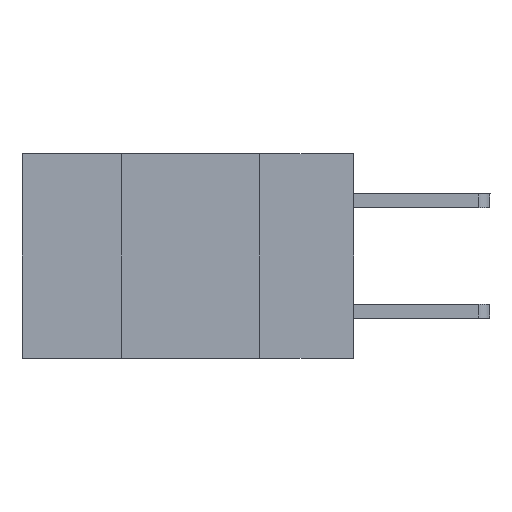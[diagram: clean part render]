
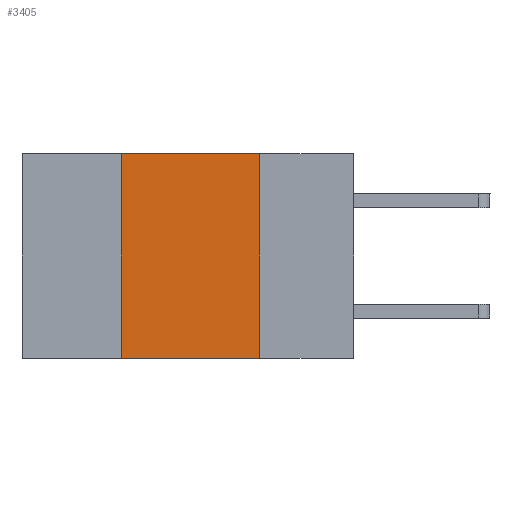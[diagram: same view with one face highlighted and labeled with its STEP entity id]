
A CAD part, left-side view. The second image highlights one B-rep face of the part: STEP entity #3405.
In plain terms, the highlighted planar face has unit normal (-1, 0, 0).
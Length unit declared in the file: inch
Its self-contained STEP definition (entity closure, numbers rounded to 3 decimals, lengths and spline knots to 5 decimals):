
#118 = EDGE_CURVE ( 'NONE', #2263, #1840, #2727, .T. ) ;
#458 = EDGE_CURVE ( 'NONE', #1840, #5806, #6440, .T. ) ;
#470 = CARTESIAN_POINT ( 'NONE',  ( 0., 0.42, -0.37 ) ) ;
#482 = DIRECTION ( 'NONE',  ( 0., 0., -1. ) ) ;
#914 = ORIENTED_EDGE ( 'NONE', *, *, #118, .F. ) ;
#1840 = VERTEX_POINT ( 'NONE', #5349 ) ;
#2181 = CARTESIAN_POINT ( 'NONE',  ( 0., 0.6, 0. ) ) ;
#2190 = ORIENTED_EDGE ( 'NONE', *, *, #10138, .T. ) ;
#2263 = VERTEX_POINT ( 'NONE', #5125 ) ;
#2301 = VECTOR ( 'NONE', #12396, 39.37008 ) ;
#2376 = ORIENTED_EDGE ( 'NONE', *, *, #9378, .F. ) ;
#2727 = LINE ( 'NONE', #11437, #2301 ) ;
#2927 = DIRECTION ( 'NONE',  ( 0., 0., -1. ) ) ;
#3405 = ADVANCED_FACE ( 'NONE', ( #5164 ), #8704, .F. ) ;
#4052 = VERTEX_POINT ( 'NONE', #470 ) ;
#4908 = DIRECTION ( 'NONE',  ( 1., 0., 0. ) ) ;
#5125 = CARTESIAN_POINT ( 'NONE',  ( 0., 0.42, 0. ) ) ;
#5164 = FACE_OUTER_BOUND ( 'NONE', #12755, .T. ) ;
#5349 = CARTESIAN_POINT ( 'NONE',  ( 0., 0.17, 0. ) ) ;
#5586 = DIRECTION ( 'NONE',  ( 0., -1., 0. ) ) ;
#5806 = VERTEX_POINT ( 'NONE', #5840 ) ;
#5808 = VECTOR ( 'NONE', #482, 39.37008 ) ;
#5815 = DIRECTION ( 'NONE',  ( 0., 0., 1. ) ) ;
#5840 = CARTESIAN_POINT ( 'NONE',  ( 0., 0.17, -0.37 ) ) ;
#6390 = VECTOR ( 'NONE', #5586, 39.37008 ) ;
#6440 = LINE ( 'NONE', #9325, #5808 ) ;
#6509 = CARTESIAN_POINT ( 'NONE',  ( 0., 0.6, -0.37 ) ) ;
#7633 = AXIS2_PLACEMENT_3D ( 'NONE', #2181, #4908, #2927 ) ;
#7977 = ORIENTED_EDGE ( 'NONE', *, *, #458, .F. ) ;
#8704 = PLANE ( 'NONE',  #7633 ) ;
#9325 = CARTESIAN_POINT ( 'NONE',  ( 0., 0.17, 0. ) ) ;
#9378 = EDGE_CURVE ( 'NONE', #4052, #2263, #12577, .T. ) ;
#9635 = CARTESIAN_POINT ( 'NONE',  ( 0., 0.42, 0. ) ) ;
#10138 = EDGE_CURVE ( 'NONE', #4052, #5806, #11641, .T. ) ;
#10887 = VECTOR ( 'NONE', #5815, 39.37008 ) ;
#11437 = CARTESIAN_POINT ( 'NONE',  ( 0., 0.6, 0. ) ) ;
#11641 = LINE ( 'NONE', #6509, #6390 ) ;
#12396 = DIRECTION ( 'NONE',  ( 0., -1., 0. ) ) ;
#12577 = LINE ( 'NONE', #9635, #10887 ) ;
#12755 = EDGE_LOOP ( 'NONE', ( #7977, #914, #2376, #2190 ) ) ;
